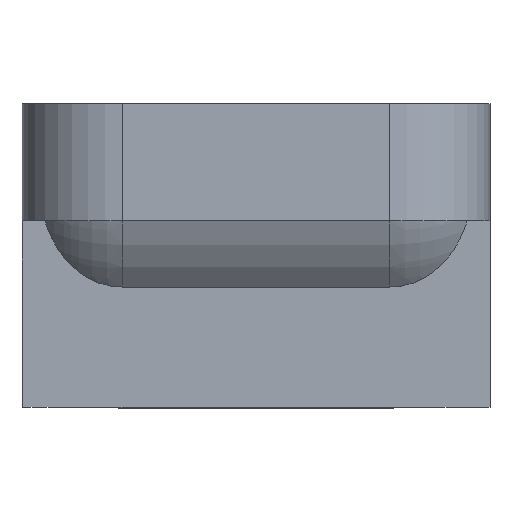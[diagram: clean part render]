
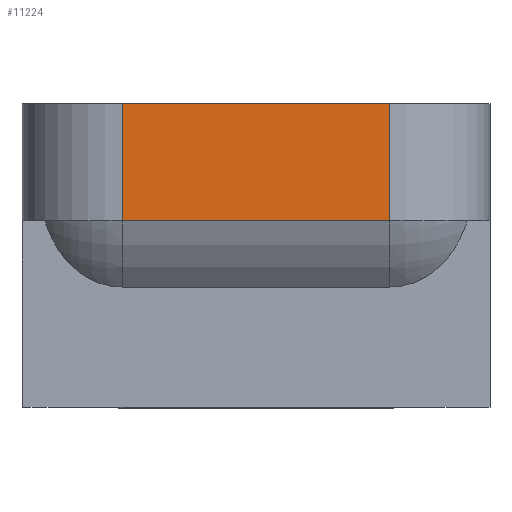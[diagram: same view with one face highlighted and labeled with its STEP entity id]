
A CAD part, front view. The second image highlights one B-rep face of the part: STEP entity #11224.
In plain terms, the highlighted planar face has unit normal (0, -1, 0).
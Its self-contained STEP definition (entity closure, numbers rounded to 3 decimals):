
#2357 = PLANE('',#2358);
#2358 = AXIS2_PLACEMENT_3D('',#2359,#2360,#2361);
#2359 = CARTESIAN_POINT('',(-7.,-8.5,-2.4));
#2360 = DIRECTION('',(0.,0.,1.));
#2361 = DIRECTION('',(0.,1.,0.));
#6923 = EDGE_CURVE('',#6924,#6926,#6928,.T.);
#6924 = VERTEX_POINT('',#6925);
#6925 = CARTESIAN_POINT('',(-4.,-8.5,-2.4));
#6926 = VERTEX_POINT('',#6927);
#6927 = CARTESIAN_POINT('',(4.,-8.5,-2.4));
#6928 = SURFACE_CURVE('',#6929,(#6933,#6940),.PCURVE_S1.);
#6929 = LINE('',#6930,#6931);
#6930 = CARTESIAN_POINT('',(-7.,-8.5,-2.4));
#6931 = VECTOR('',#6932,1.);
#6932 = DIRECTION('',(1.,0.,0.));
#6933 = PCURVE('',#2357,#6934);
#6934 = DEFINITIONAL_REPRESENTATION('',(#6935),#6939);
#6935 = LINE('',#6936,#6937);
#6936 = CARTESIAN_POINT('',(0.,0.));
#6937 = VECTOR('',#6938,1.);
#6938 = DIRECTION('',(0.,-1.));
#6939 = ( GEOMETRIC_REPRESENTATION_CONTEXT(2) 
PARAMETRIC_REPRESENTATION_CONTEXT() REPRESENTATION_CONTEXT('2D SPACE',''
  ) );
#6940 = PCURVE('',#6941,#6946);
#6941 = PLANE('',#6942);
#6942 = AXIS2_PLACEMENT_3D('',#6943,#6944,#6945);
#6943 = CARTESIAN_POINT('',(-7.,-8.5,1.1));
#6944 = DIRECTION('',(0.,1.,0.));
#6945 = DIRECTION('',(0.,0.,-1.));
#6946 = DEFINITIONAL_REPRESENTATION('',(#6947),#6951);
#6947 = LINE('',#6948,#6949);
#6948 = CARTESIAN_POINT('',(3.5,0.));
#6949 = VECTOR('',#6950,1.);
#6950 = DIRECTION('',(0.,-1.));
#6951 = ( GEOMETRIC_REPRESENTATION_CONTEXT(2) 
PARAMETRIC_REPRESENTATION_CONTEXT() REPRESENTATION_CONTEXT('2D SPACE',''
  ) );
#6970 = CYLINDRICAL_SURFACE('',#6971,3.);
#6971 = AXIS2_PLACEMENT_3D('',#6972,#6973,#6974);
#6972 = CARTESIAN_POINT('',(4.,-5.5,1.1));
#6973 = DIRECTION('',(0.,0.,-1.));
#6974 = DIRECTION('',(0.,-1.,0.));
#7786 = CYLINDRICAL_SURFACE('',#7787,3.);
#7787 = AXIS2_PLACEMENT_3D('',#7788,#7789,#7790);
#7788 = CARTESIAN_POINT('',(-4.,-5.5,1.1));
#7789 = DIRECTION('',(0.,0.,-1.));
#7790 = DIRECTION('',(-1.,0.,0.));
#9833 = PLANE('',#9834);
#9834 = AXIS2_PLACEMENT_3D('',#9835,#9836,#9837);
#9835 = CARTESIAN_POINT('',(-7.,4.,1.1));
#9836 = DIRECTION('',(0.,0.,-1.));
#9837 = DIRECTION('',(0.,-1.,0.));
#11224 = ADVANCED_FACE('',(#11225),#6941,.F.);
#11225 = FACE_BOUND('',#11226,.F.);
#11226 = EDGE_LOOP('',(#11227,#11252,#11273,#11274));
#11227 = ORIENTED_EDGE('',*,*,#11228,.T.);
#11228 = EDGE_CURVE('',#11229,#11231,#11233,.T.);
#11229 = VERTEX_POINT('',#11230);
#11230 = CARTESIAN_POINT('',(-4.,-8.5,1.1));
#11231 = VERTEX_POINT('',#11232);
#11232 = CARTESIAN_POINT('',(4.,-8.5,1.1));
#11233 = SURFACE_CURVE('',#11234,(#11238,#11245),.PCURVE_S1.);
#11234 = LINE('',#11235,#11236);
#11235 = CARTESIAN_POINT('',(-7.,-8.5,1.1));
#11236 = VECTOR('',#11237,1.);
#11237 = DIRECTION('',(1.,0.,0.));
#11238 = PCURVE('',#6941,#11239);
#11239 = DEFINITIONAL_REPRESENTATION('',(#11240),#11244);
#11240 = LINE('',#11241,#11242);
#11241 = CARTESIAN_POINT('',(0.,0.));
#11242 = VECTOR('',#11243,1.);
#11243 = DIRECTION('',(0.,-1.));
#11244 = ( GEOMETRIC_REPRESENTATION_CONTEXT(2) 
PARAMETRIC_REPRESENTATION_CONTEXT() REPRESENTATION_CONTEXT('2D SPACE',''
  ) );
#11245 = PCURVE('',#9833,#11246);
#11246 = DEFINITIONAL_REPRESENTATION('',(#11247),#11251);
#11247 = LINE('',#11248,#11249);
#11248 = CARTESIAN_POINT('',(12.5,0.));
#11249 = VECTOR('',#11250,1.);
#11250 = DIRECTION('',(0.,-1.));
#11251 = ( GEOMETRIC_REPRESENTATION_CONTEXT(2) 
PARAMETRIC_REPRESENTATION_CONTEXT() REPRESENTATION_CONTEXT('2D SPACE',''
  ) );
#11252 = ORIENTED_EDGE('',*,*,#11253,.T.);
#11253 = EDGE_CURVE('',#11231,#6926,#11254,.T.);
#11254 = SURFACE_CURVE('',#11255,(#11259,#11266),.PCURVE_S1.);
#11255 = LINE('',#11256,#11257);
#11256 = CARTESIAN_POINT('',(4.,-8.5,1.1));
#11257 = VECTOR('',#11258,1.);
#11258 = DIRECTION('',(0.,0.,-1.));
#11259 = PCURVE('',#6941,#11260);
#11260 = DEFINITIONAL_REPRESENTATION('',(#11261),#11265);
#11261 = LINE('',#11262,#11263);
#11262 = CARTESIAN_POINT('',(0.,-11.));
#11263 = VECTOR('',#11264,1.);
#11264 = DIRECTION('',(1.,0.));
#11265 = ( GEOMETRIC_REPRESENTATION_CONTEXT(2) 
PARAMETRIC_REPRESENTATION_CONTEXT() REPRESENTATION_CONTEXT('2D SPACE',''
  ) );
#11266 = PCURVE('',#6970,#11267);
#11267 = DEFINITIONAL_REPRESENTATION('',(#11268),#11272);
#11268 = LINE('',#11269,#11270);
#11269 = CARTESIAN_POINT('',(0.,0.));
#11270 = VECTOR('',#11271,1.);
#11271 = DIRECTION('',(0.,1.));
#11272 = ( GEOMETRIC_REPRESENTATION_CONTEXT(2) 
PARAMETRIC_REPRESENTATION_CONTEXT() REPRESENTATION_CONTEXT('2D SPACE',''
  ) );
#11273 = ORIENTED_EDGE('',*,*,#6923,.F.);
#11274 = ORIENTED_EDGE('',*,*,#11275,.F.);
#11275 = EDGE_CURVE('',#11229,#6924,#11276,.T.);
#11276 = SURFACE_CURVE('',#11277,(#11281,#11288),.PCURVE_S1.);
#11277 = LINE('',#11278,#11279);
#11278 = CARTESIAN_POINT('',(-4.,-8.5,1.1));
#11279 = VECTOR('',#11280,1.);
#11280 = DIRECTION('',(0.,0.,-1.));
#11281 = PCURVE('',#6941,#11282);
#11282 = DEFINITIONAL_REPRESENTATION('',(#11283),#11287);
#11283 = LINE('',#11284,#11285);
#11284 = CARTESIAN_POINT('',(0.,-3.));
#11285 = VECTOR('',#11286,1.);
#11286 = DIRECTION('',(1.,0.));
#11287 = ( GEOMETRIC_REPRESENTATION_CONTEXT(2) 
PARAMETRIC_REPRESENTATION_CONTEXT() REPRESENTATION_CONTEXT('2D SPACE',''
  ) );
#11288 = PCURVE('',#7786,#11289);
#11289 = DEFINITIONAL_REPRESENTATION('',(#11290),#11294);
#11290 = LINE('',#11291,#11292);
#11291 = CARTESIAN_POINT('',(-1.571,0.));
#11292 = VECTOR('',#11293,1.);
#11293 = DIRECTION('',(0.,1.));
#11294 = ( GEOMETRIC_REPRESENTATION_CONTEXT(2) 
PARAMETRIC_REPRESENTATION_CONTEXT() REPRESENTATION_CONTEXT('2D SPACE',''
  ) );
